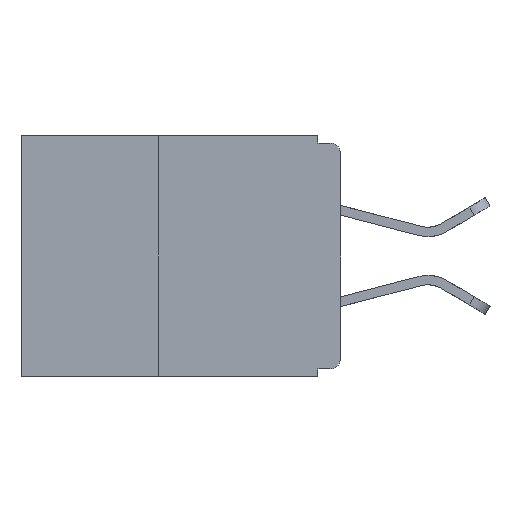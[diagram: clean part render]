
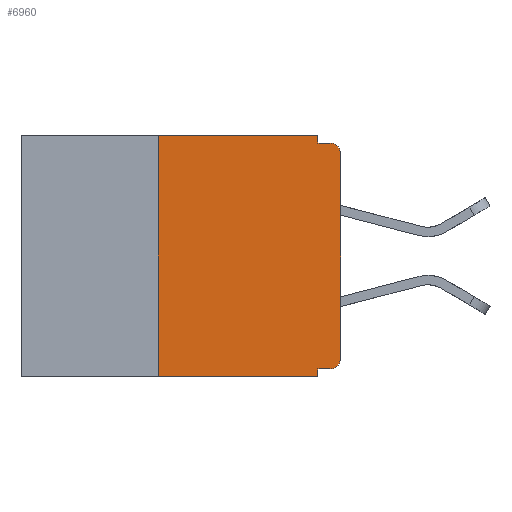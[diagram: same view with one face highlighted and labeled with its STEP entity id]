
A CAD part, left-side view. The second image highlights one B-rep face of the part: STEP entity #6960.
In plain terms, the highlighted planar face has unit normal (-1, 0, 0).
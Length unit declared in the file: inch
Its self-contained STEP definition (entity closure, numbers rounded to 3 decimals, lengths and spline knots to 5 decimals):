
#167 = DIRECTION ( 'NONE',  ( 1., 0., 0. ) ) ;
#515 = VERTEX_POINT ( 'NONE', #2156 ) ;
#561 = ORIENTED_EDGE ( 'NONE', *, *, #9169, .F. ) ;
#1045 = CARTESIAN_POINT ( 'NONE',  ( 0., 0., -0.01 ) ) ;
#1053 = CARTESIAN_POINT ( 'NONE',  ( 0., 0.031, 0. ) ) ;
#1123 = CARTESIAN_POINT ( 'NONE',  ( 0., 0.015, -0.025 ) ) ;
#1417 = CARTESIAN_POINT ( 'NONE',  ( 0., 0., -0.305 ) ) ;
#1445 = EDGE_CURVE ( 'NONE', #7140, #7015, #4607, .T. ) ;
#1800 = LINE ( 'NONE', #2228, #7582 ) ;
#2156 = CARTESIAN_POINT ( 'NONE',  ( 0., 0.031, -0.32 ) ) ;
#2178 = DIRECTION ( 'NONE',  ( 0., -1., 0. ) ) ;
#2228 = CARTESIAN_POINT ( 'NONE',  ( 0., 0.437, 0. ) ) ;
#2283 = EDGE_CURVE ( 'NONE', #7015, #7923, #2575, .T. ) ;
#2287 = DIRECTION ( 'NONE',  ( 0., 0., -1. ) ) ;
#2302 = VECTOR ( 'NONE', #11350, 39.37008 ) ;
#2309 = AXIS2_PLACEMENT_3D ( 'NONE', #9525, #9295, #4492 ) ;
#2335 = ORIENTED_EDGE ( 'NONE', *, *, #7445, .F. ) ;
#2575 = LINE ( 'NONE', #14734, #10984 ) ;
#2675 = ORIENTED_EDGE ( 'NONE', *, *, #14157, .F. ) ;
#3178 = ORIENTED_EDGE ( 'NONE', *, *, #6553, .T. ) ;
#3477 = ORIENTED_EDGE ( 'NONE', *, *, #3960, .F. ) ;
#3678 = EDGE_CURVE ( 'NONE', #4485, #12929, #1800, .T. ) ;
#3721 = CARTESIAN_POINT ( 'NONE',  ( 0., 0.25, -0.33 ) ) ;
#3725 = ORIENTED_EDGE ( 'NONE', *, *, #1445, .T. ) ;
#3920 = EDGE_CURVE ( 'NONE', #8233, #7202, #10757, .T. ) ;
#3960 = EDGE_CURVE ( 'NONE', #7140, #515, #7030, .T. ) ;
#3997 = VECTOR ( 'NONE', #13320, 39.37008 ) ;
#4038 = VECTOR ( 'NONE', #5506, 39.37008 ) ;
#4136 = ORIENTED_EDGE ( 'NONE', *, *, #3678, .F. ) ;
#4198 = CARTESIAN_POINT ( 'NONE',  ( 0., 0.437, -0.33 ) ) ;
#4485 = VERTEX_POINT ( 'NONE', #6331 ) ;
#4492 = DIRECTION ( 'NONE',  ( 0., 0., -1. ) ) ;
#4607 = CIRCLE ( 'NONE', #2309, 0.015 ) ;
#4974 = LINE ( 'NONE', #1053, #7662 ) ;
#4995 = CARTESIAN_POINT ( 'NONE',  ( 0., 0.25, -0.33 ) ) ;
#5230 = EDGE_LOOP ( 'NONE', ( #6990, #3178, #9108, #2335, #4136, #2675, #14309, #561, #3477, #3725 ) ) ;
#5356 = VERTEX_POINT ( 'NONE', #6968 ) ;
#5506 = DIRECTION ( 'NONE',  ( 0., 0., -1. ) ) ;
#5916 = PLANE ( 'NONE',  #14208 ) ;
#6331 = CARTESIAN_POINT ( 'NONE',  ( 0., 0.25, 0. ) ) ;
#6553 = EDGE_CURVE ( 'NONE', #7923, #7057, #8239, .T. ) ;
#6803 = DIRECTION ( 'NONE',  ( 0., 0., -1. ) ) ;
#6960 = ADVANCED_FACE ( 'NONE', ( #9975 ), #5916, .F. ) ;
#6968 = CARTESIAN_POINT ( 'NONE',  ( 0., 0.031, -0.01 ) ) ;
#6990 = ORIENTED_EDGE ( 'NONE', *, *, #2283, .T. ) ;
#7015 = VERTEX_POINT ( 'NONE', #1417 ) ;
#7030 = LINE ( 'NONE', #13278, #3997 ) ;
#7057 = VERTEX_POINT ( 'NONE', #7277 ) ;
#7140 = VERTEX_POINT ( 'NONE', #13096 ) ;
#7202 = VERTEX_POINT ( 'NONE', #10925 ) ;
#7277 = CARTESIAN_POINT ( 'NONE',  ( 0., 0.015, -0.01 ) ) ;
#7445 = EDGE_CURVE ( 'NONE', #12929, #5356, #4974, .T. ) ;
#7582 = VECTOR ( 'NONE', #2178, 39.37008 ) ;
#7662 = VECTOR ( 'NONE', #6803, 39.37008 ) ;
#7923 = VERTEX_POINT ( 'NONE', #13466 ) ;
#8228 = DIRECTION ( 'NONE',  ( 0., 0., -1. ) ) ;
#8233 = VERTEX_POINT ( 'NONE', #4995 ) ;
#8239 = CIRCLE ( 'NONE', #9200, 0.015 ) ;
#9108 = ORIENTED_EDGE ( 'NONE', *, *, #11653, .F. ) ;
#9166 = DIRECTION ( 'NONE',  ( -1., 0., 0. ) ) ;
#9169 = EDGE_CURVE ( 'NONE', #515, #7202, #10086, .T. ) ;
#9200 = AXIS2_PLACEMENT_3D ( 'NONE', #1123, #9166, #2287 ) ;
#9295 = DIRECTION ( 'NONE',  ( -1., 0., 0. ) ) ;
#9525 = CARTESIAN_POINT ( 'NONE',  ( 0., 0.015, -0.305 ) ) ;
#9975 = FACE_OUTER_BOUND ( 'NONE', #5230, .T. ) ;
#10086 = LINE ( 'NONE', #13427, #4038 ) ;
#10757 = LINE ( 'NONE', #4198, #13385 ) ;
#10925 = CARTESIAN_POINT ( 'NONE',  ( 0., 0.031, -0.33 ) ) ;
#10984 = VECTOR ( 'NONE', #14645, 39.37008 ) ;
#11205 = LINE ( 'NONE', #3721, #14192 ) ;
#11350 = DIRECTION ( 'NONE',  ( 0., -1., 0. ) ) ;
#11653 = EDGE_CURVE ( 'NONE', #5356, #7057, #14776, .T. ) ;
#12139 = DIRECTION ( 'NONE',  ( 0., -1., 0. ) ) ;
#12797 = DIRECTION ( 'NONE',  ( 0., 0., 1. ) ) ;
#12929 = VERTEX_POINT ( 'NONE', #14012 ) ;
#13096 = CARTESIAN_POINT ( 'NONE',  ( 0., 0.015, -0.32 ) ) ;
#13278 = CARTESIAN_POINT ( 'NONE',  ( 0., 0., -0.32 ) ) ;
#13320 = DIRECTION ( 'NONE',  ( 0., 1., 0. ) ) ;
#13385 = VECTOR ( 'NONE', #12139, 39.37008 ) ;
#13427 = CARTESIAN_POINT ( 'NONE',  ( 0., 0.031, -0.33 ) ) ;
#13466 = CARTESIAN_POINT ( 'NONE',  ( 0., 0., -0.025 ) ) ;
#13837 = CARTESIAN_POINT ( 'NONE',  ( 0., 0.437, 0. ) ) ;
#14012 = CARTESIAN_POINT ( 'NONE',  ( 0., 0.031, 0. ) ) ;
#14157 = EDGE_CURVE ( 'NONE', #8233, #4485, #11205, .T. ) ;
#14192 = VECTOR ( 'NONE', #12797, 39.37008 ) ;
#14208 = AXIS2_PLACEMENT_3D ( 'NONE', #13837, #167, #8228 ) ;
#14309 = ORIENTED_EDGE ( 'NONE', *, *, #3920, .T. ) ;
#14645 = DIRECTION ( 'NONE',  ( 0., 0., 1. ) ) ;
#14734 = CARTESIAN_POINT ( 'NONE',  ( 0., 0., 0. ) ) ;
#14776 = LINE ( 'NONE', #1045, #2302 ) ;
